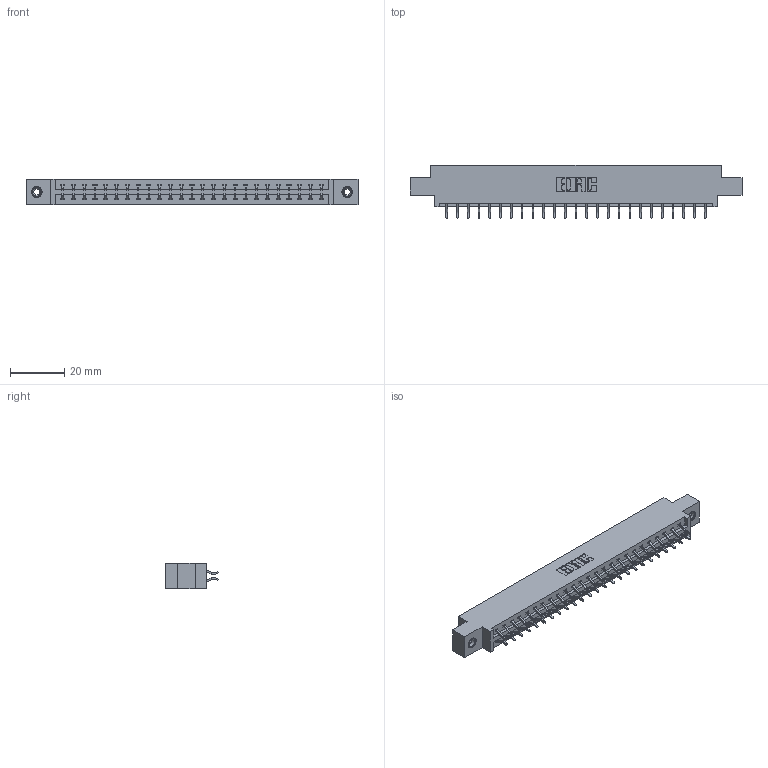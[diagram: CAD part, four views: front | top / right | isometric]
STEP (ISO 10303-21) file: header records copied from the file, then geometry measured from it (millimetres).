
FILE_DESCRIPTION (( 'STEP AP203' ), '1' );
FILE_NAME ('387-050-556-808.STEP', '2019-10-19T02:21:34', ( '' ), ( '' ), 'SwSTEP 2.0', 'SolidWorks 2016', '' );
FILE_SCHEMA (( 'CONFIG_CONTROL_DESIGN' ));
Length unit declared in the file: inch
Products named in the file (4): 345-292-001_556 Tail; 387-050-556-808; 337 Part_0.170 Offset - 0.156 Dia-TI; 345-250-001_345-250-003-102
Assembly tree (53 placements, depth 2):
  387-050-556-808
    337 Part_0.170 Offset - 0.156 Dia-TI
    345-292-001_556 Tail  x50
    345-250-001_345-250-003-102  x2
Bounding box: 122.07 x 19.57 x 9.4 mm (x, y, z)
Volume: 12512.7 mm3; surface area: 14059.5 mm2
Topology: 53 solids, 53 shells, 3178 faces, 9409 edges, 6198 vertices
Faces by surface type: plane 2206, cylinder 956, cone 12, torus 4
Entity records: 23120 total; most frequent: CARTESIAN_POINT 3905, ORIENTED_EDGE 3822, DIRECTION 3373, EDGE_CURVE 1911, LINE 1755, VECTOR 1755, VERTEX_POINT 1268, AXIS2_PLACEMENT_3D 809
